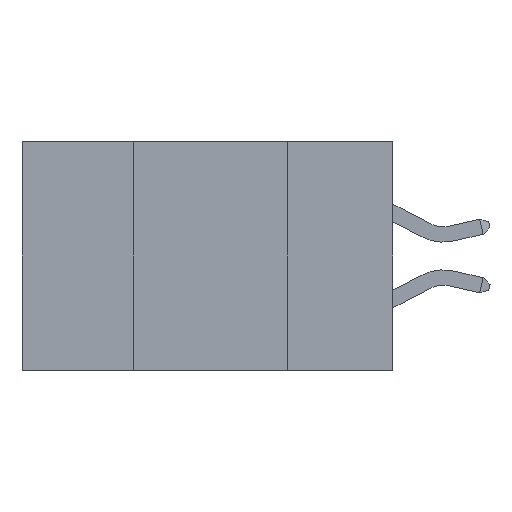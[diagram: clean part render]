
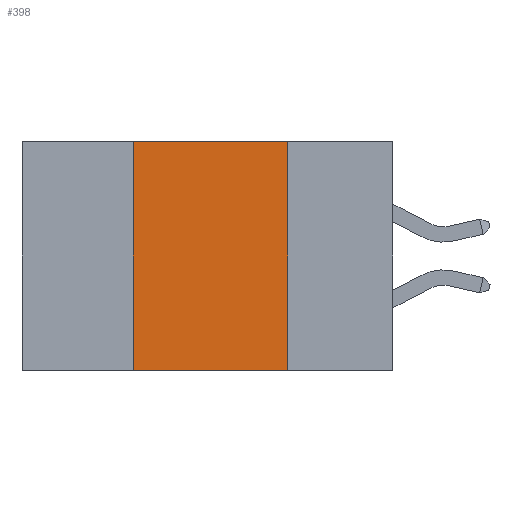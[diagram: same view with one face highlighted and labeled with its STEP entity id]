
A CAD part, left-side view. The second image highlights one B-rep face of the part: STEP entity #398.
In plain terms, the highlighted planar face has unit normal (-1, 0, 0).
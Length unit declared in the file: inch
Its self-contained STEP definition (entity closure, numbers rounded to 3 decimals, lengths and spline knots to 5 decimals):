
#241 = DIRECTION ( 'NONE',  ( 0., -1., 0. ) ) ;
#398 = ADVANCED_FACE ( 'NONE', ( #7550 ), #6290, .F. ) ;
#525 = EDGE_LOOP ( 'NONE', ( #11698, #2203, #890, #3297 ) ) ;
#890 = ORIENTED_EDGE ( 'NONE', *, *, #2009, .F. ) ;
#1011 = LINE ( 'NONE', #2468, #4509 ) ;
#1163 = VECTOR ( 'NONE', #2830, 39.37008 ) ;
#1487 = VERTEX_POINT ( 'NONE', #10437 ) ;
#2009 = EDGE_CURVE ( 'NONE', #12265, #1487, #8206, .T. ) ;
#2145 = CARTESIAN_POINT ( 'NONE',  ( 0., 0.42, -0.37 ) ) ;
#2203 = ORIENTED_EDGE ( 'NONE', *, *, #9401, .F. ) ;
#2468 = CARTESIAN_POINT ( 'NONE',  ( 0., 0.6, 0. ) ) ;
#2830 = DIRECTION ( 'NONE',  ( 0., 0., -1. ) ) ;
#3169 = DIRECTION ( 'NONE',  ( 0., 0., 1. ) ) ;
#3297 = ORIENTED_EDGE ( 'NONE', *, *, #7317, .T. ) ;
#3835 = LINE ( 'NONE', #12366, #1163 ) ;
#4509 = VECTOR ( 'NONE', #4668, 39.37008 ) ;
#4668 = DIRECTION ( 'NONE',  ( 0., -1., 0. ) ) ;
#4671 = CARTESIAN_POINT ( 'NONE',  ( 0., 0.6, -0.37 ) ) ;
#5072 = EDGE_CURVE ( 'NONE', #11378, #9370, #3835, .T. ) ;
#5190 = DIRECTION ( 'NONE',  ( 0., 0., -1. ) ) ;
#5796 = CARTESIAN_POINT ( 'NONE',  ( 0., 0.17, -0.37 ) ) ;
#6290 = PLANE ( 'NONE',  #8192 ) ;
#6374 = DIRECTION ( 'NONE',  ( 1., 0., 0. ) ) ;
#6461 = CARTESIAN_POINT ( 'NONE',  ( 0., 0.42, 0. ) ) ;
#6921 = VECTOR ( 'NONE', #241, 39.37008 ) ;
#7317 = EDGE_CURVE ( 'NONE', #12265, #9370, #9273, .T. ) ;
#7550 = FACE_OUTER_BOUND ( 'NONE', #525, .T. ) ;
#8192 = AXIS2_PLACEMENT_3D ( 'NONE', #13761, #6374, #5190 ) ;
#8206 = LINE ( 'NONE', #6461, #13578 ) ;
#9273 = LINE ( 'NONE', #4671, #6921 ) ;
#9370 = VERTEX_POINT ( 'NONE', #5796 ) ;
#9401 = EDGE_CURVE ( 'NONE', #1487, #11378, #1011, .T. ) ;
#10437 = CARTESIAN_POINT ( 'NONE',  ( 0., 0.42, 0. ) ) ;
#11378 = VERTEX_POINT ( 'NONE', #13251 ) ;
#11698 = ORIENTED_EDGE ( 'NONE', *, *, #5072, .F. ) ;
#12265 = VERTEX_POINT ( 'NONE', #2145 ) ;
#12366 = CARTESIAN_POINT ( 'NONE',  ( 0., 0.17, 0. ) ) ;
#13251 = CARTESIAN_POINT ( 'NONE',  ( 0., 0.17, 0. ) ) ;
#13578 = VECTOR ( 'NONE', #3169, 39.37008 ) ;
#13761 = CARTESIAN_POINT ( 'NONE',  ( 0., 0.6, 0. ) ) ;
